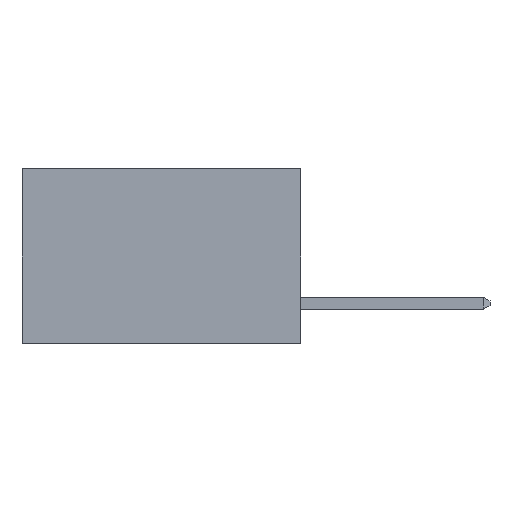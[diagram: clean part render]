
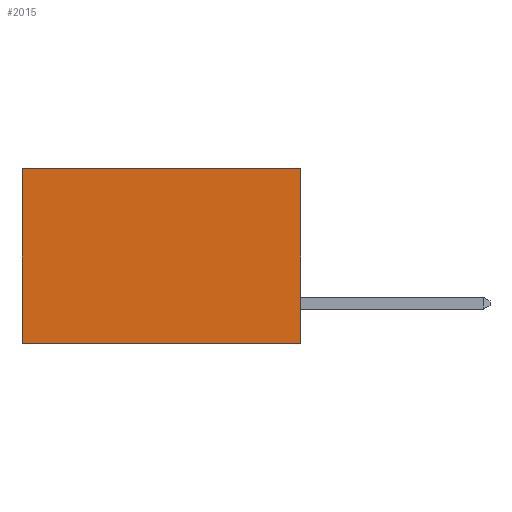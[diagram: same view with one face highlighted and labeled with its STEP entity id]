
A CAD part, left-side view. The second image highlights one B-rep face of the part: STEP entity #2015.
In plain terms, the highlighted planar face has unit normal (-1, 0, 0).
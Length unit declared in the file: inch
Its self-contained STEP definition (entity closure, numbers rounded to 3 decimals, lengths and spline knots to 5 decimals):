
#90 = LINE ( 'NONE', #240, #8907 ) ;
#240 = CARTESIAN_POINT ( 'NONE',  ( 0.277, 0.59, -0.37 ) ) ;
#426 = DIRECTION ( 'NONE',  ( 0., 0., -1. ) ) ;
#658 = VERTEX_POINT ( 'NONE', #8053 ) ;
#1226 = VECTOR ( 'NONE', #2284, 39.37008 ) ;
#1427 = FACE_OUTER_BOUND ( 'NONE', #9544, .T. ) ;
#1789 = EDGE_CURVE ( 'NONE', #4222, #5285, #9301, .T. ) ;
#2015 = ADVANCED_FACE ( 'NONE', ( #1427 ), #9265, .F. ) ;
#2047 = VECTOR ( 'NONE', #9569, 39.37008 ) ;
#2225 = EDGE_CURVE ( 'NONE', #8527, #658, #90, .T. ) ;
#2248 = CARTESIAN_POINT ( 'NONE',  ( 0.277, 0., -0.37 ) ) ;
#2258 = CARTESIAN_POINT ( 'NONE',  ( 0.277, 0., 0. ) ) ;
#2284 = DIRECTION ( 'NONE',  ( 0., 1., 0. ) ) ;
#2925 = EDGE_CURVE ( 'NONE', #4222, #8527, #3538, .T. ) ;
#3515 = DIRECTION ( 'NONE',  ( 0., 0., -1. ) ) ;
#3538 = LINE ( 'NONE', #2258, #1226 ) ;
#3998 = CARTESIAN_POINT ( 'NONE',  ( 0.277, 0.59, 0. ) ) ;
#4222 = VERTEX_POINT ( 'NONE', #7789 ) ;
#4259 = DIRECTION ( 'NONE',  ( 0., 0., -1. ) ) ;
#5249 = CARTESIAN_POINT ( 'NONE',  ( 0.277, 0., -0.37 ) ) ;
#5285 = VERTEX_POINT ( 'NONE', #5249 ) ;
#6709 = CARTESIAN_POINT ( 'NONE',  ( 0.277, 0., -0.37 ) ) ;
#7617 = VECTOR ( 'NONE', #3515, 39.37008 ) ;
#7789 = CARTESIAN_POINT ( 'NONE',  ( 0.277, 0., 0. ) ) ;
#7937 = CARTESIAN_POINT ( 'NONE',  ( 0.277, 0., -0.37 ) ) ;
#8053 = CARTESIAN_POINT ( 'NONE',  ( 0.277, 0.59, -0.37 ) ) ;
#8081 = ORIENTED_EDGE ( 'NONE', *, *, #2225, .T. ) ;
#8390 = ORIENTED_EDGE ( 'NONE', *, *, #10287, .F. ) ;
#8400 = ORIENTED_EDGE ( 'NONE', *, *, #1789, .F. ) ;
#8527 = VERTEX_POINT ( 'NONE', #3998 ) ;
#8636 = ORIENTED_EDGE ( 'NONE', *, *, #2925, .T. ) ;
#8907 = VECTOR ( 'NONE', #426, 39.37008 ) ;
#9187 = DIRECTION ( 'NONE',  ( 1., 0., 0. ) ) ;
#9265 = PLANE ( 'NONE',  #9867 ) ;
#9301 = LINE ( 'NONE', #2248, #7617 ) ;
#9544 = EDGE_LOOP ( 'NONE', ( #8081, #8390, #8400, #8636 ) ) ;
#9569 = DIRECTION ( 'NONE',  ( 0., 1., 0. ) ) ;
#9867 = AXIS2_PLACEMENT_3D ( 'NONE', #6709, #9187, #4259 ) ;
#10287 = EDGE_CURVE ( 'NONE', #5285, #658, #10539, .T. ) ;
#10539 = LINE ( 'NONE', #7937, #2047 ) ;
